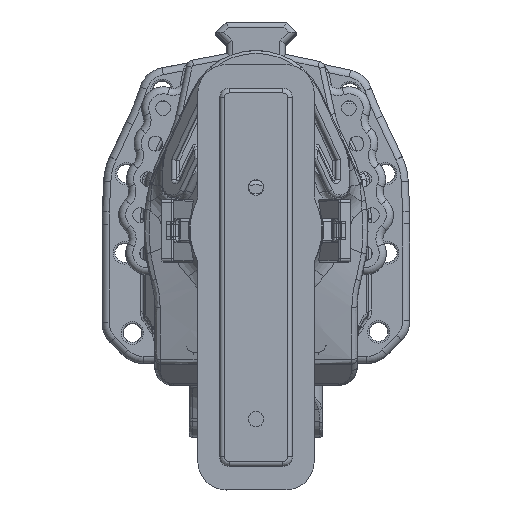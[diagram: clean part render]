
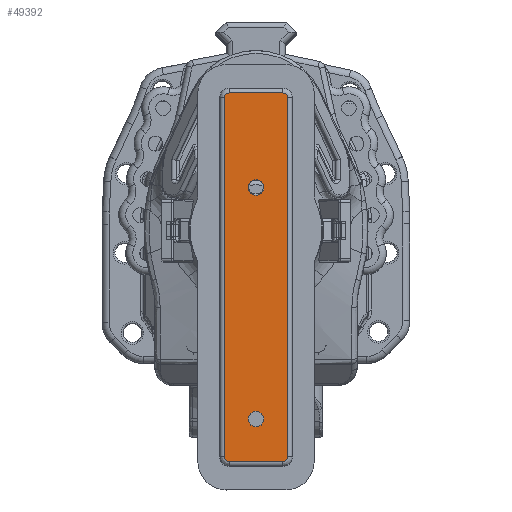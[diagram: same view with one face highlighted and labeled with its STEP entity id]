
A CAD part, top view. The second image highlights one B-rep face of the part: STEP entity #49392.
In plain terms, the highlighted face is planar.
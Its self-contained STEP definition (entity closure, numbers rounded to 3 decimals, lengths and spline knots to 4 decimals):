
#374=FACE_BOUND('',#9072,.T.);
#375=FACE_BOUND('',#9073,.T.);
#1628=PLANE('',#54585);
#6062=FACE_OUTER_BOUND('',#9071,.T.);
#9071=EDGE_LOOP('',(#44088,#44089,#44090,#44091,#44092,#44093,#44094,#44095));
#9072=EDGE_LOOP('',(#44096,#44097));
#9073=EDGE_LOOP('',(#44098,#44099));
#12717=LINE('',#101035,#16374);
#12718=LINE('',#101041,#16375);
#12719=LINE('',#101045,#16376);
#12720=LINE('',#101050,#16377);
#16374=VECTOR('',#67727,0.3937);
#16375=VECTOR('',#67734,0.3937);
#16376=VECTOR('',#67737,0.3937);
#16377=VECTOR('',#67742,0.3937);
#18662=CIRCLE('',#54204,0.0827);
#18663=CIRCLE('',#54205,0.0827);
#18665=CIRCLE('',#54208,0.0827);
#18666=CIRCLE('',#54209,0.0827);
#18868=CIRCLE('',#54586,0.05);
#18869=CIRCLE('',#54587,0.05);
#18870=CIRCLE('',#54588,0.05);
#18871=CIRCLE('',#54589,0.05);
#22939=VERTEX_POINT('',#98450);
#22940=VERTEX_POINT('',#98451);
#22942=VERTEX_POINT('',#98458);
#22943=VERTEX_POINT('',#98459);
#23287=VERTEX_POINT('',#101033);
#23288=VERTEX_POINT('',#101034);
#23289=VERTEX_POINT('',#101039);
#23290=VERTEX_POINT('',#101040);
#23291=VERTEX_POINT('',#101042);
#23292=VERTEX_POINT('',#101044);
#23293=VERTEX_POINT('',#101047);
#23294=VERTEX_POINT('',#101049);
#29793=EDGE_CURVE('',#22939,#22940,#18662,.T.);
#29794=EDGE_CURVE('',#22940,#22939,#18663,.T.);
#29797=EDGE_CURVE('',#22942,#22943,#18665,.T.);
#29798=EDGE_CURVE('',#22943,#22942,#18666,.T.);
#30303=EDGE_CURVE('',#23287,#23288,#12717,.T.);
#30306=EDGE_CURVE('',#23289,#23290,#12718,.T.);
#30307=EDGE_CURVE('',#23291,#23289,#18868,.T.);
#30308=EDGE_CURVE('',#23292,#23291,#12719,.T.);
#30309=EDGE_CURVE('',#23288,#23292,#18869,.T.);
#30310=EDGE_CURVE('',#23293,#23287,#18870,.T.);
#30311=EDGE_CURVE('',#23294,#23293,#12720,.T.);
#30312=EDGE_CURVE('',#23290,#23294,#18871,.T.);
#44088=ORIENTED_EDGE('',*,*,#30306,.F.);
#44089=ORIENTED_EDGE('',*,*,#30307,.F.);
#44090=ORIENTED_EDGE('',*,*,#30308,.F.);
#44091=ORIENTED_EDGE('',*,*,#30309,.F.);
#44092=ORIENTED_EDGE('',*,*,#30303,.F.);
#44093=ORIENTED_EDGE('',*,*,#30310,.F.);
#44094=ORIENTED_EDGE('',*,*,#30311,.F.);
#44095=ORIENTED_EDGE('',*,*,#30312,.F.);
#44096=ORIENTED_EDGE('',*,*,#29793,.T.);
#44097=ORIENTED_EDGE('',*,*,#29794,.T.);
#44098=ORIENTED_EDGE('',*,*,#29797,.T.);
#44099=ORIENTED_EDGE('',*,*,#29798,.T.);
#49392=ADVANCED_FACE('',(#6062,#374,#375),#1628,.T.);
#54204=AXIS2_PLACEMENT_3D('',#98452,#66790,#66791);
#54205=AXIS2_PLACEMENT_3D('',#98453,#66792,#66793);
#54208=AXIS2_PLACEMENT_3D('',#98460,#66799,#66800);
#54209=AXIS2_PLACEMENT_3D('',#98461,#66801,#66802);
#54585=AXIS2_PLACEMENT_3D('',#101038,#67732,#67733);
#54586=AXIS2_PLACEMENT_3D('',#101043,#67735,#67736);
#54587=AXIS2_PLACEMENT_3D('',#101046,#67738,#67739);
#54588=AXIS2_PLACEMENT_3D('',#101048,#67740,#67741);
#54589=AXIS2_PLACEMENT_3D('',#101051,#67743,#67744);
#66790=DIRECTION('center_axis',(-1.,0.,0.));
#66791=DIRECTION('ref_axis',(0.,0.,-1.));
#66792=DIRECTION('center_axis',(-1.,0.,0.));
#66793=DIRECTION('ref_axis',(0.,0.,-1.));
#66799=DIRECTION('center_axis',(-1.,0.,0.));
#66800=DIRECTION('ref_axis',(0.,0.,-1.));
#66801=DIRECTION('center_axis',(-1.,0.,0.));
#66802=DIRECTION('ref_axis',(0.,0.,-1.));
#67727=DIRECTION('',(0.,-1.,0.));
#67732=DIRECTION('center_axis',(1.,0.,0.));
#67733=DIRECTION('ref_axis',(0.,0.,-1.));
#67734=DIRECTION('',(0.,1.,0.));
#67735=DIRECTION('center_axis',(-1.,0.,0.));
#67736=DIRECTION('ref_axis',(0.,-0.707,0.707));
#67737=DIRECTION('',(0.,0.,1.));
#67738=DIRECTION('center_axis',(-1.,0.,0.));
#67739=DIRECTION('ref_axis',(0.,-0.707,-0.707));
#67740=DIRECTION('center_axis',(-1.,0.,0.));
#67741=DIRECTION('ref_axis',(0.,0.707,-0.707));
#67742=DIRECTION('',(0.,0.,-1.));
#67743=DIRECTION('center_axis',(-1.,0.,0.));
#67744=DIRECTION('ref_axis',(0.,0.707,0.707));
#98450=CARTESIAN_POINT('',(6.64,-2.1,-0.0827));
#98451=CARTESIAN_POINT('',(6.64,-2.1,0.0827));
#98452=CARTESIAN_POINT('Origin',(6.64,-2.1,0.));
#98453=CARTESIAN_POINT('Origin',(6.64,-2.1,0.));
#98458=CARTESIAN_POINT('',(6.64,0.35,-0.0827));
#98459=CARTESIAN_POINT('',(6.64,0.35,0.0827));
#98460=CARTESIAN_POINT('Origin',(6.64,0.35,0.));
#98461=CARTESIAN_POINT('Origin',(6.64,0.35,0.));
#101033=CARTESIAN_POINT('',(6.64,1.3,-0.335));
#101034=CARTESIAN_POINT('',(6.64,-2.5,-0.335));
#101035=CARTESIAN_POINT('',(6.64,-1.55,-0.335));
#101038=CARTESIAN_POINT('Origin',(6.64,-0.6,0.));
#101039=CARTESIAN_POINT('',(6.64,-2.5,0.335));
#101040=CARTESIAN_POINT('',(6.64,1.3,0.335));
#101041=CARTESIAN_POINT('',(6.64,0.35,0.335));
#101042=CARTESIAN_POINT('',(6.64,-2.55,0.285));
#101043=CARTESIAN_POINT('Origin',(6.64,-2.5,0.285));
#101044=CARTESIAN_POINT('',(6.64,-2.55,-0.285));
#101045=CARTESIAN_POINT('',(6.64,-2.55,0.1425));
#101046=CARTESIAN_POINT('Origin',(6.64,-2.5,-0.285));
#101047=CARTESIAN_POINT('',(6.64,1.35,-0.285));
#101048=CARTESIAN_POINT('Origin',(6.64,1.3,-0.285));
#101049=CARTESIAN_POINT('',(6.64,1.35,0.285));
#101050=CARTESIAN_POINT('',(6.64,1.35,-0.1425));
#101051=CARTESIAN_POINT('Origin',(6.64,1.3,0.285));
